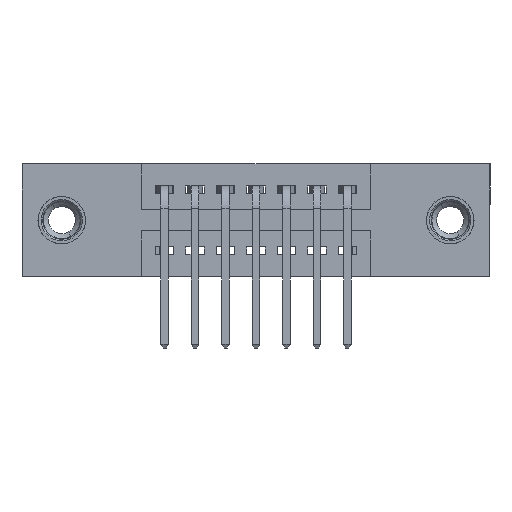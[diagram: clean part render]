
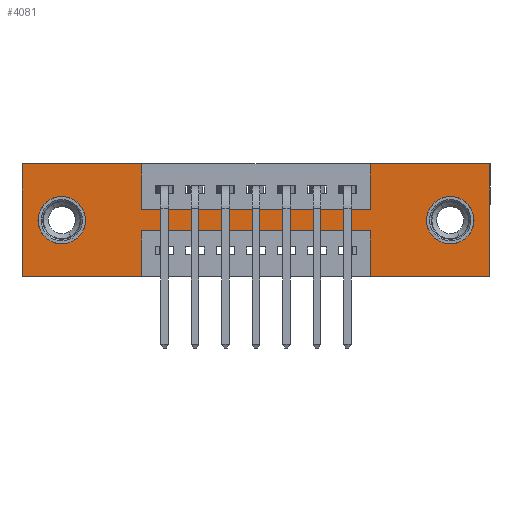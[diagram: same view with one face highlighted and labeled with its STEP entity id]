
A CAD part, front view. The second image highlights one B-rep face of the part: STEP entity #4081.
In plain terms, the highlighted planar face has unit normal (0, -1, 0).
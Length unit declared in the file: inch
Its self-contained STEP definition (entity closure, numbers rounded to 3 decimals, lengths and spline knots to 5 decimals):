
#141 = EDGE_CURVE ( 'NONE', #8632, #6947, #8436, .T. ) ;
#296 = CARTESIAN_POINT ( 'NONE',  ( 0.3925, 0., 0. ) ) ;
#399 = VECTOR ( 'NONE', #6047, 39.37008 ) ;
#661 = DIRECTION ( 'NONE',  ( 0., 0., -1. ) ) ;
#694 = EDGE_CURVE ( 'NONE', #10285, #14756, #10760, .T. ) ;
#1020 = VERTEX_POINT ( 'NONE', #1527 ) ;
#1031 = ORIENTED_EDGE ( 'NONE', *, *, #11849, .F. ) ;
#1087 = CARTESIAN_POINT ( 'NONE',  ( 0.13, 0., -0.185 ) ) ;
#1116 = CARTESIAN_POINT ( 'NONE',  ( 1.1425, 0., -0.22 ) ) ;
#1152 = EDGE_CURVE ( 'NONE', #4575, #3844, #11100, .T. ) ;
#1452 = CARTESIAN_POINT ( 'NONE',  ( 1.1425, 0., -0.37 ) ) ;
#1495 = CARTESIAN_POINT ( 'NONE',  ( 1.535, 0., 0. ) ) ;
#1527 = CARTESIAN_POINT ( 'NONE',  ( 0.13, 0., -0.263 ) ) ;
#1775 = CIRCLE ( 'NONE', #2300, 0.078 ) ;
#1823 = DIRECTION ( 'NONE',  ( 0., 1., 0. ) ) ;
#1855 = LINE ( 'NONE', #4432, #13650 ) ;
#1858 = EDGE_CURVE ( 'NONE', #4854, #7999, #8372, .T. ) ;
#1986 = CARTESIAN_POINT ( 'NONE',  ( 0., 0., -0.37 ) ) ;
#2032 = ORIENTED_EDGE ( 'NONE', *, *, #694, .F. ) ;
#2068 = DIRECTION ( 'NONE',  ( 1., 0., 0. ) ) ;
#2237 = CARTESIAN_POINT ( 'NONE',  ( 0.3925, 0., -0.37 ) ) ;
#2246 = DIRECTION ( 'NONE',  ( 0., 0., 1. ) ) ;
#2273 = VERTEX_POINT ( 'NONE', #1452 ) ;
#2300 = AXIS2_PLACEMENT_3D ( 'NONE', #5091, #13086, #6242 ) ;
#2409 = FACE_BOUND ( 'NONE', #2838, .T. ) ;
#2420 = LINE ( 'NONE', #13468, #7783 ) ;
#2742 = ORIENTED_EDGE ( 'NONE', *, *, #13760, .T. ) ;
#2838 = EDGE_LOOP ( 'NONE', ( #12732, #9241 ) ) ;
#3171 = DIRECTION ( 'NONE',  ( 0., 0., 1. ) ) ;
#3275 = VERTEX_POINT ( 'NONE', #7151 ) ;
#3343 = DIRECTION ( 'NONE',  ( 0., 0., 1. ) ) ;
#3524 = ORIENTED_EDGE ( 'NONE', *, *, #13334, .F. ) ;
#3568 = VECTOR ( 'NONE', #10257, 39.37008 ) ;
#3574 = ORIENTED_EDGE ( 'NONE', *, *, #1152, .F. ) ;
#3656 = EDGE_CURVE ( 'NONE', #2273, #10285, #2420, .T. ) ;
#3657 = CARTESIAN_POINT ( 'NONE',  ( 1.535, 0., 0. ) ) ;
#3736 = AXIS2_PLACEMENT_3D ( 'NONE', #6358, #7519, #661 ) ;
#3794 = CIRCLE ( 'NONE', #5486, 0.078 ) ;
#3816 = CARTESIAN_POINT ( 'NONE',  ( 1.1425, 0., 0. ) ) ;
#3844 = VERTEX_POINT ( 'NONE', #7078 ) ;
#4081 = ADVANCED_FACE ( 'NONE', ( #2409, #5440, #14205 ), #14350, .T. ) ;
#4088 = DIRECTION ( 'NONE',  ( -1., 0., 0. ) ) ;
#4154 = CARTESIAN_POINT ( 'NONE',  ( 0., 0., 0. ) ) ;
#4259 = EDGE_LOOP ( 'NONE', ( #13779, #2742 ) ) ;
#4268 = VECTOR ( 'NONE', #2068, 39.37008 ) ;
#4329 = EDGE_CURVE ( 'NONE', #13707, #8632, #1855, .T. ) ;
#4431 = VERTEX_POINT ( 'NONE', #8119 ) ;
#4432 = CARTESIAN_POINT ( 'NONE',  ( 1.1425, 0., 0. ) ) ;
#4470 = AXIS2_PLACEMENT_3D ( 'NONE', #9019, #9132, #14031 ) ;
#4474 = CARTESIAN_POINT ( 'NONE',  ( 1.535, 0., -0.37 ) ) ;
#4575 = VERTEX_POINT ( 'NONE', #5103 ) ;
#4671 = LINE ( 'NONE', #4900, #10433 ) ;
#4687 = VECTOR ( 'NONE', #14271, 39.37008 ) ;
#4854 = VERTEX_POINT ( 'NONE', #14582 ) ;
#4900 = CARTESIAN_POINT ( 'NONE',  ( 0., 0., 0. ) ) ;
#4934 = VERTEX_POINT ( 'NONE', #4474 ) ;
#4944 = EDGE_CURVE ( 'NONE', #11156, #1020, #3794, .T. ) ;
#5091 = CARTESIAN_POINT ( 'NONE',  ( 1.405, 0., -0.185 ) ) ;
#5103 = CARTESIAN_POINT ( 'NONE',  ( 0.3925, 0., -0.37 ) ) ;
#5104 = ORIENTED_EDGE ( 'NONE', *, *, #12334, .F. ) ;
#5382 = EDGE_CURVE ( 'NONE', #4431, #9125, #6839, .T. ) ;
#5419 = LINE ( 'NONE', #6228, #4687 ) ;
#5440 = FACE_BOUND ( 'NONE', #4259, .T. ) ;
#5453 = CARTESIAN_POINT ( 'NONE',  ( 0.13, 0., -0.107 ) ) ;
#5486 = AXIS2_PLACEMENT_3D ( 'NONE', #1087, #9117, #2246 ) ;
#5978 = CARTESIAN_POINT ( 'NONE',  ( 0., 0., -0.37 ) ) ;
#6047 = DIRECTION ( 'NONE',  ( 0., 0., -1. ) ) ;
#6228 = CARTESIAN_POINT ( 'NONE',  ( 0.3925, 0., 0. ) ) ;
#6242 = DIRECTION ( 'NONE',  ( 0., 0., -1. ) ) ;
#6358 = CARTESIAN_POINT ( 'NONE',  ( 0., 0., -0.37 ) ) ;
#6586 = DIRECTION ( 'NONE',  ( -1., 0., 0. ) ) ;
#6839 = LINE ( 'NONE', #4154, #7205 ) ;
#6947 = VERTEX_POINT ( 'NONE', #3657 ) ;
#7078 = CARTESIAN_POINT ( 'NONE',  ( 0., 0., -0.37 ) ) ;
#7084 = ORIENTED_EDGE ( 'NONE', *, *, #10994, .F. ) ;
#7151 = CARTESIAN_POINT ( 'NONE',  ( 0.3925, 0., -0.15 ) ) ;
#7168 = AXIS2_PLACEMENT_3D ( 'NONE', #8678, #1823, #9845 ) ;
#7205 = VECTOR ( 'NONE', #12179, 39.37008 ) ;
#7267 = ORIENTED_EDGE ( 'NONE', *, *, #3656, .F. ) ;
#7344 = EDGE_CURVE ( 'NONE', #3275, #13707, #7347, .T. ) ;
#7347 = LINE ( 'NONE', #7725, #4268 ) ;
#7355 = VECTOR ( 'NONE', #8823, 39.37008 ) ;
#7429 = CARTESIAN_POINT ( 'NONE',  ( 1.1425, 0., -0.15 ) ) ;
#7519 = DIRECTION ( 'NONE',  ( 0., -1., 0. ) ) ;
#7725 = CARTESIAN_POINT ( 'NONE',  ( 0.3925, 0., -0.15 ) ) ;
#7783 = VECTOR ( 'NONE', #3171, 39.37008 ) ;
#7952 = EDGE_LOOP ( 'NONE', ( #3524, #2032, #7267, #10205, #7084, #9479, #10430, #9981, #1031, #10790, #5104, #3574 ) ) ;
#7999 = VERTEX_POINT ( 'NONE', #13935 ) ;
#8119 = CARTESIAN_POINT ( 'NONE',  ( 0., 0., 0. ) ) ;
#8124 = EDGE_CURVE ( 'NONE', #7999, #4854, #1775, .T. ) ;
#8337 = EDGE_CURVE ( 'NONE', #4934, #2273, #13381, .T. ) ;
#8372 = CIRCLE ( 'NONE', #4470, 0.078 ) ;
#8418 = CARTESIAN_POINT ( 'NONE',  ( 0.3925, 0., -0.22 ) ) ;
#8436 = LINE ( 'NONE', #8453, #14147 ) ;
#8453 = CARTESIAN_POINT ( 'NONE',  ( 0., 0., 0. ) ) ;
#8632 = VERTEX_POINT ( 'NONE', #3816 ) ;
#8678 = CARTESIAN_POINT ( 'NONE',  ( 0.13, 0., -0.185 ) ) ;
#8823 = DIRECTION ( 'NONE',  ( -1., 0., 0. ) ) ;
#9019 = CARTESIAN_POINT ( 'NONE',  ( 1.405, 0., -0.185 ) ) ;
#9117 = DIRECTION ( 'NONE',  ( 0., 1., 0. ) ) ;
#9125 = VERTEX_POINT ( 'NONE', #296 ) ;
#9132 = DIRECTION ( 'NONE',  ( 0., 1., 0. ) ) ;
#9241 = ORIENTED_EDGE ( 'NONE', *, *, #1858, .T. ) ;
#9479 = ORIENTED_EDGE ( 'NONE', *, *, #141, .F. ) ;
#9845 = DIRECTION ( 'NONE',  ( 0., 0., 1. ) ) ;
#9981 = ORIENTED_EDGE ( 'NONE', *, *, #7344, .F. ) ;
#10034 = CIRCLE ( 'NONE', #7168, 0.078 ) ;
#10185 = CARTESIAN_POINT ( 'NONE',  ( 0.3925, 0., -0.22 ) ) ;
#10205 = ORIENTED_EDGE ( 'NONE', *, *, #8337, .F. ) ;
#10257 = DIRECTION ( 'NONE',  ( 0., 0., -1. ) ) ;
#10285 = VERTEX_POINT ( 'NONE', #1116 ) ;
#10301 = DIRECTION ( 'NONE',  ( 1., 0., 0. ) ) ;
#10380 = VECTOR ( 'NONE', #6586, 39.37008 ) ;
#10430 = ORIENTED_EDGE ( 'NONE', *, *, #4329, .F. ) ;
#10433 = VECTOR ( 'NONE', #14055, 39.37008 ) ;
#10760 = LINE ( 'NONE', #8418, #7355 ) ;
#10790 = ORIENTED_EDGE ( 'NONE', *, *, #5382, .F. ) ;
#10994 = EDGE_CURVE ( 'NONE', #6947, #4934, #11507, .T. ) ;
#11100 = LINE ( 'NONE', #5978, #13403 ) ;
#11156 = VERTEX_POINT ( 'NONE', #5453 ) ;
#11507 = LINE ( 'NONE', #1495, #399 ) ;
#11849 = EDGE_CURVE ( 'NONE', #9125, #3275, #5419, .T. ) ;
#12179 = DIRECTION ( 'NONE',  ( 1., 0., 0. ) ) ;
#12334 = EDGE_CURVE ( 'NONE', #3844, #4431, #4671, .T. ) ;
#12732 = ORIENTED_EDGE ( 'NONE', *, *, #8124, .T. ) ;
#13066 = LINE ( 'NONE', #2237, #3568 ) ;
#13086 = DIRECTION ( 'NONE',  ( 0., 1., 0. ) ) ;
#13334 = EDGE_CURVE ( 'NONE', #14756, #4575, #13066, .T. ) ;
#13381 = LINE ( 'NONE', #1986, #10380 ) ;
#13403 = VECTOR ( 'NONE', #4088, 39.37008 ) ;
#13468 = CARTESIAN_POINT ( 'NONE',  ( 1.1425, 0., -0.37 ) ) ;
#13650 = VECTOR ( 'NONE', #3343, 39.37008 ) ;
#13707 = VERTEX_POINT ( 'NONE', #7429 ) ;
#13760 = EDGE_CURVE ( 'NONE', #1020, #11156, #10034, .T. ) ;
#13779 = ORIENTED_EDGE ( 'NONE', *, *, #4944, .T. ) ;
#13935 = CARTESIAN_POINT ( 'NONE',  ( 1.405, 0., -0.107 ) ) ;
#14031 = DIRECTION ( 'NONE',  ( 0., 0., -1. ) ) ;
#14055 = DIRECTION ( 'NONE',  ( 0., 0., 1. ) ) ;
#14147 = VECTOR ( 'NONE', #10301, 39.37008 ) ;
#14205 = FACE_OUTER_BOUND ( 'NONE', #7952, .T. ) ;
#14271 = DIRECTION ( 'NONE',  ( 0., 0., -1. ) ) ;
#14350 = PLANE ( 'NONE',  #3736 ) ;
#14582 = CARTESIAN_POINT ( 'NONE',  ( 1.405, 0., -0.263 ) ) ;
#14756 = VERTEX_POINT ( 'NONE', #10185 ) ;
